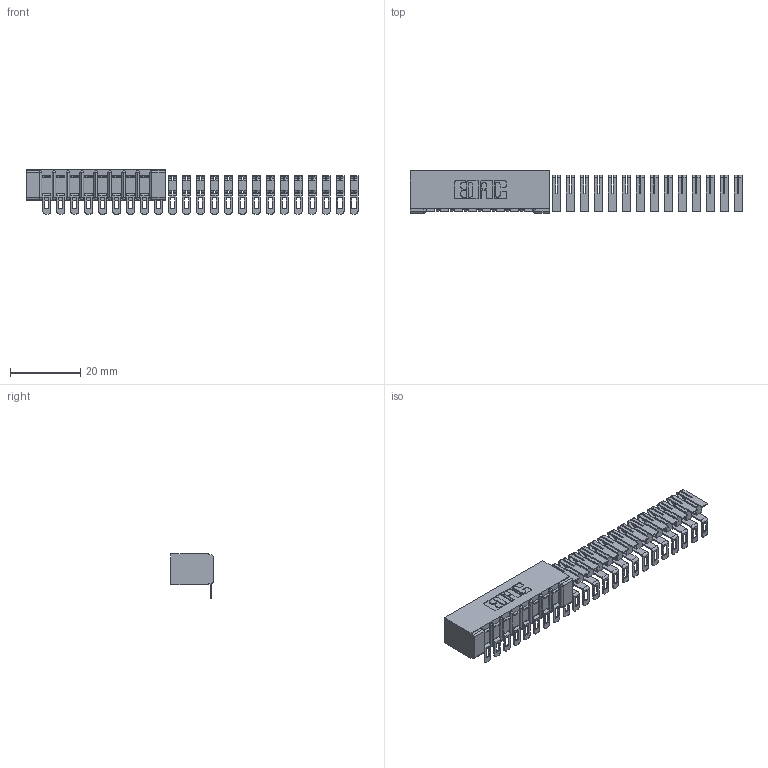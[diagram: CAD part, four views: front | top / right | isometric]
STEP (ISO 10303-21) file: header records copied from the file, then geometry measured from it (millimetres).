
FILE_DESCRIPTION (( 'STEP AP203' ), '1' );
FILE_NAME ('357-023-554-101.STEP', '2018-08-08T23:50:04', ( '' ), ( '' ), 'SwSTEP 2.0', 'SolidWorks 2016', '' );
FILE_SCHEMA (( 'CONFIG_CONTROL_DESIGN' ));
Length unit declared in the file: inch
Products named in the file (3): 307 Part_No Mounting Lugs; 307-290-002_554; 357-023-554-101
Assembly tree (24 placements, depth 2):
  357-023-554-101
    307 Part_No Mounting Lugs
    307-290-002_554  x23
Bounding box: 94.22 x 12.01 x 12.52 mm (x, y, z)
Volume: 3289.9 mm3; surface area: 8336.7 mm2
Topology: 24 solids, 24 shells, 1682 faces, 5158 edges, 3412 vertices
Faces by surface type: plane 944, cylinder 720, sphere 18
Entity records: 12217 total; most frequent: CARTESIAN_POINT 1989, DIRECTION 1968, ORIENTED_EDGE 1964, EDGE_CURVE 982, LINE 730, VECTOR 730, VERTEX_POINT 640, AXIS2_PLACEMENT_3D 619
